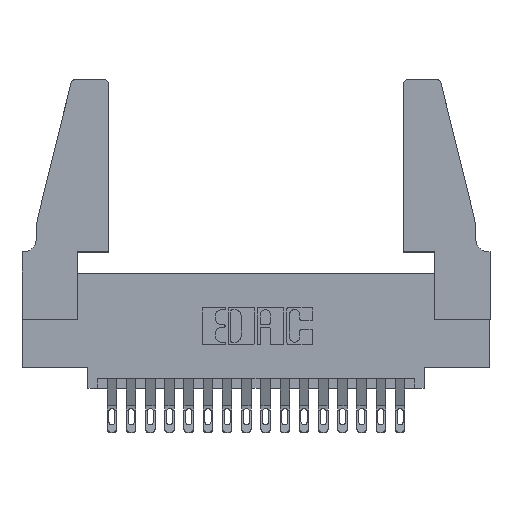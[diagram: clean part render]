
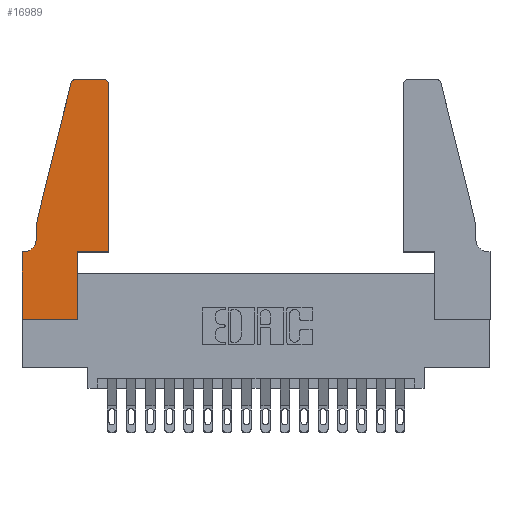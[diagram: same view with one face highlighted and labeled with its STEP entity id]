
A CAD part, top view. The second image highlights one B-rep face of the part: STEP entity #16989.
In plain terms, the highlighted planar face has unit normal (0, 0, 1).
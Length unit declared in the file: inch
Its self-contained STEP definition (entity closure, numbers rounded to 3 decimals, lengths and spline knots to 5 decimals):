
#17 = LINE ( 'NONE', #6673, #16958 ) ;
#413 = EDGE_CURVE ( 'NONE', #9889, #6546, #5243, .T. ) ;
#515 = CARTESIAN_POINT ( 'NONE',  ( 0.4505, 0.35, 0.37 ) ) ;
#537 = DIRECTION ( 'NONE',  ( 0., 0., -1. ) ) ;
#573 = VECTOR ( 'NONE', #6417, 39.37008 ) ;
#874 = DIRECTION ( 'NONE',  ( 1., 0., 0. ) ) ;
#1015 = LINE ( 'NONE', #15334, #6235 ) ;
#1250 = VECTOR ( 'NONE', #16267, 39.37008 ) ;
#1314 = DIRECTION ( 'NONE',  ( 0., 0., 1. ) ) ;
#2093 = VERTEX_POINT ( 'NONE', #18061 ) ;
#2155 = FACE_OUTER_BOUND ( 'NONE', #14995, .T. ) ;
#2389 = DIRECTION ( 'NONE',  ( -1., 0., 0. ) ) ;
#2808 = DIRECTION ( 'NONE',  ( 1., 0., 0. ) ) ;
#2976 = AXIS2_PLACEMENT_3D ( 'NONE', #10517, #4945, #17833 ) ;
#3037 = VERTEX_POINT ( 'NONE', #10828 ) ;
#3499 = ORIENTED_EDGE ( 'NONE', *, *, #9077, .T. ) ;
#3596 = VERTEX_POINT ( 'NONE', #16202 ) ;
#4021 = CARTESIAN_POINT ( 'NONE',  ( 0., 0.35, 0.37 ) ) ;
#4090 = VECTOR ( 'NONE', #6172, 39.37008 ) ;
#4147 = PLANE ( 'NONE',  #6435 ) ;
#4945 = DIRECTION ( 'NONE',  ( 0., 0., 1. ) ) ;
#4947 = ORIENTED_EDGE ( 'NONE', *, *, #15005, .T. ) ;
#5243 = CIRCLE ( 'NONE', #15643, 0.07 ) ;
#5346 = DIRECTION ( 'NONE',  ( 1., 0., 0. ) ) ;
#5529 = VECTOR ( 'NONE', #16425, 39.37008 ) ;
#5667 = VERTEX_POINT ( 'NONE', #17891 ) ;
#5759 = VERTEX_POINT ( 'NONE', #6586 ) ;
#6024 = LINE ( 'NONE', #16203, #1250 ) ;
#6068 = EDGE_CURVE ( 'NONE', #5759, #16598, #14398, .T. ) ;
#6160 = ORIENTED_EDGE ( 'NONE', *, *, #14715, .T. ) ;
#6172 = DIRECTION ( 'NONE',  ( -1., 0., 0. ) ) ;
#6235 = VECTOR ( 'NONE', #874, 39.37008 ) ;
#6287 = LINE ( 'NONE', #8466, #12112 ) ;
#6417 = DIRECTION ( 'NONE',  ( 1., 0., 0. ) ) ;
#6435 = AXIS2_PLACEMENT_3D ( 'NONE', #4021, #1314, #2808 ) ;
#6457 = ORIENTED_EDGE ( 'NONE', *, *, #7937, .T. ) ;
#6497 = VERTEX_POINT ( 'NONE', #13869 ) ;
#6546 = VERTEX_POINT ( 'NONE', #13763 ) ;
#6586 = CARTESIAN_POINT ( 'NONE',  ( 0.4205, 1.25, 0.37 ) ) ;
#6669 = ORIENTED_EDGE ( 'NONE', *, *, #8729, .T. ) ;
#6673 = CARTESIAN_POINT ( 'NONE',  ( 0.0755, 0.35, 0.37 ) ) ;
#7104 = LINE ( 'NONE', #10812, #5529 ) ;
#7111 = CARTESIAN_POINT ( 'NONE',  ( 0.0755, 0.42, 0.37 ) ) ;
#7177 = CARTESIAN_POINT ( 'NONE',  ( 0.284, 1.25, 0.37 ) ) ;
#7238 = EDGE_CURVE ( 'NONE', #16598, #3037, #9402, .T. ) ;
#7937 = EDGE_CURVE ( 'NONE', #15248, #6497, #17520, .T. ) ;
#7994 = ORIENTED_EDGE ( 'NONE', *, *, #11375, .T. ) ;
#8097 = CARTESIAN_POINT ( 'NONE',  ( 0.284, 1.22, 0.37 ) ) ;
#8355 = EDGE_CURVE ( 'NONE', #2093, #5667, #14557, .T. ) ;
#8466 = CARTESIAN_POINT ( 'NONE',  ( 0.0755, 0.5, 0.37 ) ) ;
#8729 = EDGE_CURVE ( 'NONE', #18538, #2093, #13638, .T. ) ;
#8935 = AXIS2_PLACEMENT_3D ( 'NONE', #8097, #13992, #5346 ) ;
#9038 = ORIENTED_EDGE ( 'NONE', *, *, #413, .T. ) ;
#9077 = EDGE_CURVE ( 'NONE', #5667, #3596, #7104, .T. ) ;
#9134 = VERTEX_POINT ( 'NONE', #18001 ) ;
#9295 = CARTESIAN_POINT ( 'NONE',  ( 0.2605, 1.25, 0.37 ) ) ;
#9402 = CIRCLE ( 'NONE', #8935, 0.03 ) ;
#9539 = DIRECTION ( 'NONE',  ( -1., 0., 0. ) ) ;
#9889 = VERTEX_POINT ( 'NONE', #7111 ) ;
#10024 = CARTESIAN_POINT ( 'NONE',  ( 0., 0., 0.37 ) ) ;
#10235 = ORIENTED_EDGE ( 'NONE', *, *, #6068, .T. ) ;
#10517 = CARTESIAN_POINT ( 'NONE',  ( 0.4205, 1.22, 0.37 ) ) ;
#10812 = CARTESIAN_POINT ( 'NONE',  ( 0.4505, 0.35, 0.37 ) ) ;
#10828 = CARTESIAN_POINT ( 'NONE',  ( 0.25487, 1.22718, 0.37 ) ) ;
#10839 = CIRCLE ( 'NONE', #2976, 0.03 ) ;
#11188 = VECTOR ( 'NONE', #14168, 39.37008 ) ;
#11281 = ORIENTED_EDGE ( 'NONE', *, *, #8355, .T. ) ;
#11375 = EDGE_CURVE ( 'NONE', #3596, #5759, #10839, .T. ) ;
#11935 = CARTESIAN_POINT ( 'NONE',  ( 0.0055, 0.42, 0.37 ) ) ;
#11979 = EDGE_CURVE ( 'NONE', #6546, #15248, #17, .T. ) ;
#12112 = VECTOR ( 'NONE', #18545, 39.37008 ) ;
#12189 = CARTESIAN_POINT ( 'NONE',  ( 0.2865, 0., 0.37 ) ) ;
#12717 = CARTESIAN_POINT ( 'NONE',  ( 0.2865, 0.35, 0.37 ) ) ;
#13638 = LINE ( 'NONE', #12717, #11188 ) ;
#13763 = CARTESIAN_POINT ( 'NONE',  ( 0.0055, 0.35, 0.37 ) ) ;
#13869 = CARTESIAN_POINT ( 'NONE',  ( 0., 0., 0.37 ) ) ;
#13938 = EDGE_CURVE ( 'NONE', #3037, #9134, #6287, .T. ) ;
#13992 = DIRECTION ( 'NONE',  ( 0., 0., 1. ) ) ;
#14168 = DIRECTION ( 'NONE',  ( 0., 1., 0. ) ) ;
#14316 = ORIENTED_EDGE ( 'NONE', *, *, #11979, .T. ) ;
#14398 = LINE ( 'NONE', #9295, #4090 ) ;
#14557 = LINE ( 'NONE', #515, #573 ) ;
#14715 = EDGE_CURVE ( 'NONE', #9134, #9889, #6024, .T. ) ;
#14995 = EDGE_LOOP ( 'NONE', ( #10235, #15858, #16099, #6160, #9038, #14316, #6457, #4947, #6669, #11281, #3499, #7994 ) ) ;
#15005 = EDGE_CURVE ( 'NONE', #6497, #18538, #1015, .T. ) ;
#15248 = VERTEX_POINT ( 'NONE', #17570 ) ;
#15334 = CARTESIAN_POINT ( 'NONE',  ( 0., 0., 0.37 ) ) ;
#15643 = AXIS2_PLACEMENT_3D ( 'NONE', #11935, #537, #2389 ) ;
#15858 = ORIENTED_EDGE ( 'NONE', *, *, #7238, .T. ) ;
#15876 = DIRECTION ( 'NONE',  ( 0., -1., 0. ) ) ;
#16099 = ORIENTED_EDGE ( 'NONE', *, *, #13938, .T. ) ;
#16202 = CARTESIAN_POINT ( 'NONE',  ( 0.4505, 1.22, 0.37 ) ) ;
#16203 = CARTESIAN_POINT ( 'NONE',  ( 0.0755, 0.5, 0.37 ) ) ;
#16267 = DIRECTION ( 'NONE',  ( 0., -1., 0. ) ) ;
#16425 = DIRECTION ( 'NONE',  ( 0., 1., 0. ) ) ;
#16598 = VERTEX_POINT ( 'NONE', #7177 ) ;
#16958 = VECTOR ( 'NONE', #9539, 39.37008 ) ;
#16989 = ADVANCED_FACE ( 'NONE', ( #2155 ), #4147, .T. ) ;
#17520 = LINE ( 'NONE', #10024, #17980 ) ;
#17570 = CARTESIAN_POINT ( 'NONE',  ( 0., 0.35, 0.37 ) ) ;
#17833 = DIRECTION ( 'NONE',  ( 1., 0., 0. ) ) ;
#17891 = CARTESIAN_POINT ( 'NONE',  ( 0.4505, 0.35, 0.37 ) ) ;
#17980 = VECTOR ( 'NONE', #15876, 39.37008 ) ;
#18001 = CARTESIAN_POINT ( 'NONE',  ( 0.0755, 0.5, 0.37 ) ) ;
#18061 = CARTESIAN_POINT ( 'NONE',  ( 0.2865, 0.35, 0.37 ) ) ;
#18538 = VERTEX_POINT ( 'NONE', #12189 ) ;
#18545 = DIRECTION ( 'NONE',  ( -0.239, -0.971, 0. ) ) ;
